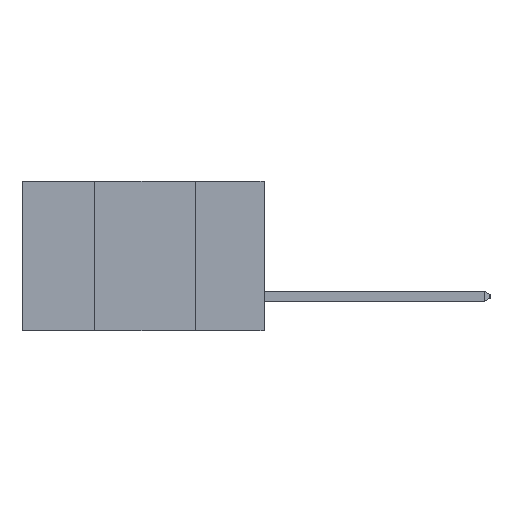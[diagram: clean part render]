
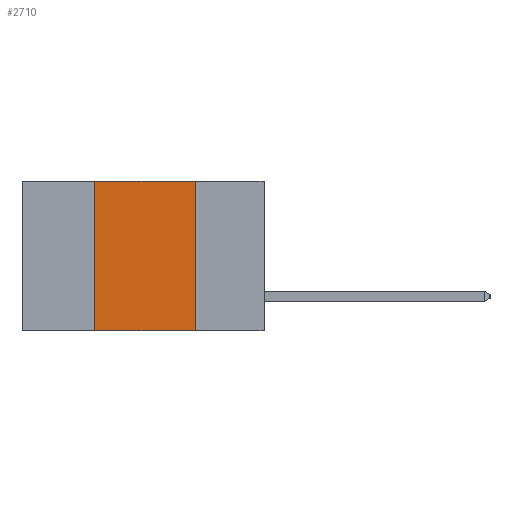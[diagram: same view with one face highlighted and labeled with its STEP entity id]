
A CAD part, left-side view. The second image highlights one B-rep face of the part: STEP entity #2710.
In plain terms, the highlighted planar face has unit normal (-1, 0, 0).
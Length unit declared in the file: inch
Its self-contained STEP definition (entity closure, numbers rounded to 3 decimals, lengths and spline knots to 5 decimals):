
#26 = LINE ( 'NONE', #552, #3632 ) ;
#130 = ORIENTED_EDGE ( 'NONE', *, *, #6434, .F. ) ;
#247 = ORIENTED_EDGE ( 'NONE', *, *, #3192, .T. ) ;
#413 = VERTEX_POINT ( 'NONE', #1744 ) ;
#552 = CARTESIAN_POINT ( 'NONE',  ( 0., 0.17, -0.37 ) ) ;
#814 = CARTESIAN_POINT ( 'NONE',  ( 0., 0.42, 0. ) ) ;
#830 = VECTOR ( 'NONE', #5163, 39.37008 ) ;
#1744 = CARTESIAN_POINT ( 'NONE',  ( 0., 0.17, -0.37 ) ) ;
#1835 = CARTESIAN_POINT ( 'NONE',  ( 0., 0.6, -0.37 ) ) ;
#2109 = LINE ( 'NONE', #5449, #4015 ) ;
#2180 = LINE ( 'NONE', #1835, #5715 ) ;
#2710 = ADVANCED_FACE ( 'NONE', ( #5725 ), #3889, .F. ) ;
#3192 = EDGE_CURVE ( 'NONE', #3300, #413, #2180, .T. ) ;
#3235 = DIRECTION ( 'NONE',  ( 0., 0., -1. ) ) ;
#3300 = VERTEX_POINT ( 'NONE', #6675 ) ;
#3395 = DIRECTION ( 'NONE',  ( 1., 0., 0. ) ) ;
#3465 = ORIENTED_EDGE ( 'NONE', *, *, #4065, .F. ) ;
#3495 = AXIS2_PLACEMENT_3D ( 'NONE', #5846, #3395, #3235 ) ;
#3632 = VECTOR ( 'NONE', #6858, 39.37008 ) ;
#3889 = PLANE ( 'NONE',  #3495 ) ;
#4015 = VECTOR ( 'NONE', #8165, 39.37008 ) ;
#4065 = EDGE_CURVE ( 'NONE', #6205, #413, #26, .T. ) ;
#4465 = ORIENTED_EDGE ( 'NONE', *, *, #8068, .F. ) ;
#5163 = DIRECTION ( 'NONE',  ( 0., -1., 0. ) ) ;
#5449 = CARTESIAN_POINT ( 'NONE',  ( 0., 0.42, -0.37 ) ) ;
#5715 = VECTOR ( 'NONE', #7194, 39.37008 ) ;
#5725 = FACE_OUTER_BOUND ( 'NONE', #6030, .T. ) ;
#5846 = CARTESIAN_POINT ( 'NONE',  ( 0., 0.6, 0. ) ) ;
#6030 = EDGE_LOOP ( 'NONE', ( #3465, #4465, #130, #247 ) ) ;
#6205 = VERTEX_POINT ( 'NONE', #6585 ) ;
#6434 = EDGE_CURVE ( 'NONE', #3300, #8703, #2109, .T. ) ;
#6469 = LINE ( 'NONE', #7848, #830 ) ;
#6585 = CARTESIAN_POINT ( 'NONE',  ( 0., 0.17, 0. ) ) ;
#6675 = CARTESIAN_POINT ( 'NONE',  ( 0., 0.42, -0.37 ) ) ;
#6858 = DIRECTION ( 'NONE',  ( 0., 0., -1. ) ) ;
#7194 = DIRECTION ( 'NONE',  ( 0., -1., 0. ) ) ;
#7848 = CARTESIAN_POINT ( 'NONE',  ( 0., 0.6, 0. ) ) ;
#8068 = EDGE_CURVE ( 'NONE', #8703, #6205, #6469, .T. ) ;
#8165 = DIRECTION ( 'NONE',  ( 0., 0., 1. ) ) ;
#8703 = VERTEX_POINT ( 'NONE', #814 ) ;
